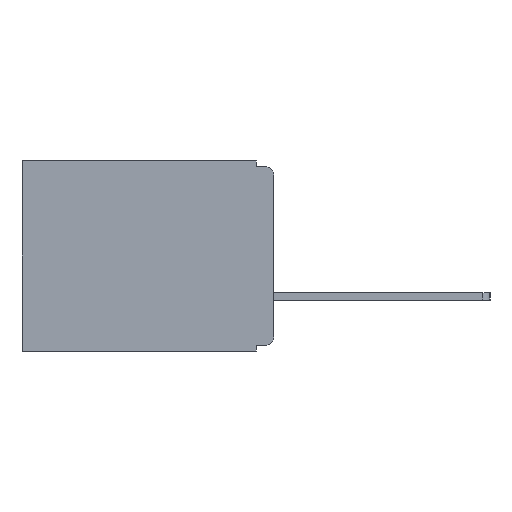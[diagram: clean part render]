
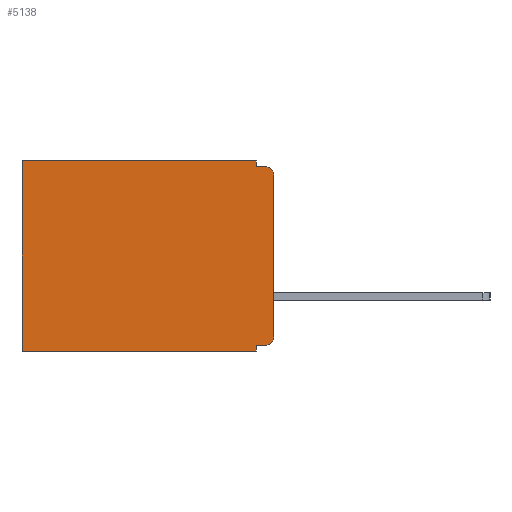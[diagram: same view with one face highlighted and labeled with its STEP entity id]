
A CAD part, left-side view. The second image highlights one B-rep face of the part: STEP entity #5138.
In plain terms, the highlighted planar face has unit normal (-1, 0, 0).
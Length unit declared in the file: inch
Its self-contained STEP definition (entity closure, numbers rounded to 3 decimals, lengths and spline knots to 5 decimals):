
#90 = DIRECTION ( 'NONE',  ( 0., 1., 0. ) ) ;
#374 = ORIENTED_EDGE ( 'NONE', *, *, #8372, .T. ) ;
#791 = VECTOR ( 'NONE', #9128, 39.37008 ) ;
#858 = CARTESIAN_POINT ( 'NONE',  ( 0.3, 0.031, -0.32 ) ) ;
#1252 = DIRECTION ( 'NONE',  ( 1., 0., 0. ) ) ;
#1366 = VECTOR ( 'NONE', #19013, 39.37008 ) ;
#1785 = VECTOR ( 'NONE', #10832, 39.37008 ) ;
#1957 = CIRCLE ( 'NONE', #2478, 0.015 ) ;
#1959 = ORIENTED_EDGE ( 'NONE', *, *, #6369, .F. ) ;
#2019 = CARTESIAN_POINT ( 'NONE',  ( 0.3, 0.015, -0.32 ) ) ;
#2205 = EDGE_CURVE ( 'NONE', #6051, #14285, #8705, .T. ) ;
#2348 = CIRCLE ( 'NONE', #3219, 0.015 ) ;
#2478 = AXIS2_PLACEMENT_3D ( 'NONE', #9617, #20778, #11285 ) ;
#2493 = ORIENTED_EDGE ( 'NONE', *, *, #20448, .T. ) ;
#2732 = VERTEX_POINT ( 'NONE', #16152 ) ;
#2836 = VERTEX_POINT ( 'NONE', #3112 ) ;
#2971 = DIRECTION ( 'NONE',  ( 0., -1., 0. ) ) ;
#3112 = CARTESIAN_POINT ( 'NONE',  ( 0.3, 0., -0.305 ) ) ;
#3219 = AXIS2_PLACEMENT_3D ( 'NONE', #15932, #6233, #17542 ) ;
#3545 = EDGE_LOOP ( 'NONE', ( #17210, #374, #17712, #5330, #13996, #10164, #1959, #10699, #14988, #2493 ) ) ;
#3549 = CARTESIAN_POINT ( 'NONE',  ( 0.3, 0.031, 0. ) ) ;
#4361 = VECTOR ( 'NONE', #6541, 39.37008 ) ;
#4422 = VERTEX_POINT ( 'NONE', #8442 ) ;
#5080 = EDGE_CURVE ( 'NONE', #6051, #16396, #17617, .T. ) ;
#5138 = ADVANCED_FACE ( 'NONE', ( #20289 ), #13116, .F. ) ;
#5330 = ORIENTED_EDGE ( 'NONE', *, *, #2205, .F. ) ;
#5675 = EDGE_CURVE ( 'NONE', #16396, #16172, #20272, .T. ) ;
#6051 = VERTEX_POINT ( 'NONE', #3549 ) ;
#6169 = LINE ( 'NONE', #11688, #1785 ) ;
#6220 = CARTESIAN_POINT ( 'NONE',  ( 0.3, 0.031, -0.01 ) ) ;
#6233 = DIRECTION ( 'NONE',  ( -1., 0., 0. ) ) ;
#6369 = EDGE_CURVE ( 'NONE', #11638, #16172, #6169, .T. ) ;
#6541 = DIRECTION ( 'NONE',  ( 0., 0., -1. ) ) ;
#6577 = CARTESIAN_POINT ( 'NONE',  ( 0.3, 0.031, 0. ) ) ;
#6970 = VECTOR ( 'NONE', #12777, 39.37008 ) ;
#7881 = CARTESIAN_POINT ( 'NONE',  ( 0.3, 0., -0.01 ) ) ;
#8372 = EDGE_CURVE ( 'NONE', #4422, #2732, #1957, .T. ) ;
#8442 = CARTESIAN_POINT ( 'NONE',  ( 0.3, 0., -0.025 ) ) ;
#8691 = LINE ( 'NONE', #19470, #4361 ) ;
#8705 = LINE ( 'NONE', #6577, #17289 ) ;
#9128 = DIRECTION ( 'NONE',  ( 0., 1., 0. ) ) ;
#9194 = CARTESIAN_POINT ( 'NONE',  ( 0.3, 0., 0. ) ) ;
#9617 = CARTESIAN_POINT ( 'NONE',  ( 0.3, 0.015, -0.025 ) ) ;
#10096 = LINE ( 'NONE', #11050, #1366 ) ;
#10164 = ORIENTED_EDGE ( 'NONE', *, *, #5675, .T. ) ;
#10347 = CARTESIAN_POINT ( 'NONE',  ( 0.3, 0.437, -0.33 ) ) ;
#10512 = DIRECTION ( 'NONE',  ( 0., 0., -1. ) ) ;
#10671 = AXIS2_PLACEMENT_3D ( 'NONE', #16903, #1252, #17324 ) ;
#10699 = ORIENTED_EDGE ( 'NONE', *, *, #11819, .F. ) ;
#10832 = DIRECTION ( 'NONE',  ( 0., 1., 0. ) ) ;
#11050 = CARTESIAN_POINT ( 'NONE',  ( 0.3, 0., -0.33 ) ) ;
#11285 = DIRECTION ( 'NONE',  ( 0., 0., -1. ) ) ;
#11638 = VERTEX_POINT ( 'NONE', #20536 ) ;
#11688 = CARTESIAN_POINT ( 'NONE',  ( 0.3, 0., -0.33 ) ) ;
#11819 = EDGE_CURVE ( 'NONE', #19255, #11638, #8691, .T. ) ;
#12704 = LINE ( 'NONE', #7881, #16931 ) ;
#12777 = DIRECTION ( 'NONE',  ( 0., 0., -1. ) ) ;
#13116 = PLANE ( 'NONE',  #10671 ) ;
#13688 = VECTOR ( 'NONE', #90, 39.37008 ) ;
#13771 = CARTESIAN_POINT ( 'NONE',  ( 0.3, 0.437, -0.33 ) ) ;
#13996 = ORIENTED_EDGE ( 'NONE', *, *, #5080, .T. ) ;
#14285 = VERTEX_POINT ( 'NONE', #6220 ) ;
#14988 = ORIENTED_EDGE ( 'NONE', *, *, #18384, .F. ) ;
#15932 = CARTESIAN_POINT ( 'NONE',  ( 0.3, 0.015, -0.305 ) ) ;
#16152 = CARTESIAN_POINT ( 'NONE',  ( 0.3, 0.015, -0.01 ) ) ;
#16172 = VERTEX_POINT ( 'NONE', #13771 ) ;
#16396 = VERTEX_POINT ( 'NONE', #19072 ) ;
#16435 = CARTESIAN_POINT ( 'NONE',  ( 0.3, 0., -0.32 ) ) ;
#16903 = CARTESIAN_POINT ( 'NONE',  ( 0.3, 0., -0.33 ) ) ;
#16931 = VECTOR ( 'NONE', #2971, 39.37008 ) ;
#17210 = ORIENTED_EDGE ( 'NONE', *, *, #18146, .F. ) ;
#17289 = VECTOR ( 'NONE', #10512, 39.37008 ) ;
#17324 = DIRECTION ( 'NONE',  ( 0., 0., -1. ) ) ;
#17542 = DIRECTION ( 'NONE',  ( 0., 0., -1. ) ) ;
#17592 = EDGE_CURVE ( 'NONE', #14285, #2732, #12704, .T. ) ;
#17617 = LINE ( 'NONE', #9194, #791 ) ;
#17712 = ORIENTED_EDGE ( 'NONE', *, *, #17592, .F. ) ;
#17858 = VERTEX_POINT ( 'NONE', #2019 ) ;
#18146 = EDGE_CURVE ( 'NONE', #4422, #2836, #10096, .T. ) ;
#18384 = EDGE_CURVE ( 'NONE', #17858, #19255, #18396, .T. ) ;
#18396 = LINE ( 'NONE', #16435, #13688 ) ;
#19013 = DIRECTION ( 'NONE',  ( 0., 0., -1. ) ) ;
#19072 = CARTESIAN_POINT ( 'NONE',  ( 0.3, 0.437, 0. ) ) ;
#19255 = VERTEX_POINT ( 'NONE', #858 ) ;
#19470 = CARTESIAN_POINT ( 'NONE',  ( 0.3, 0.031, -0.33 ) ) ;
#20272 = LINE ( 'NONE', #10347, #6970 ) ;
#20289 = FACE_OUTER_BOUND ( 'NONE', #3545, .T. ) ;
#20448 = EDGE_CURVE ( 'NONE', #17858, #2836, #2348, .T. ) ;
#20536 = CARTESIAN_POINT ( 'NONE',  ( 0.3, 0.031, -0.33 ) ) ;
#20778 = DIRECTION ( 'NONE',  ( -1., 0., 0. ) ) ;
